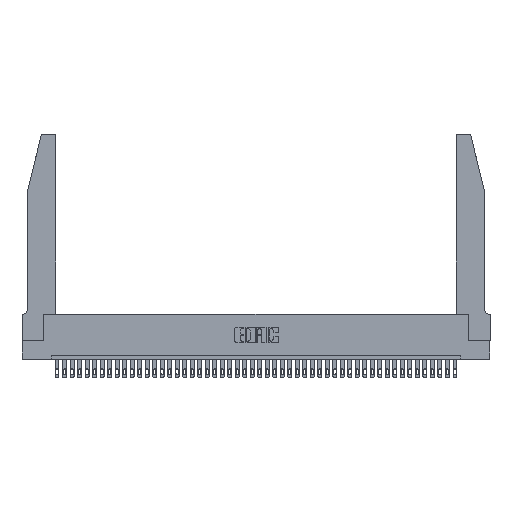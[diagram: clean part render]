
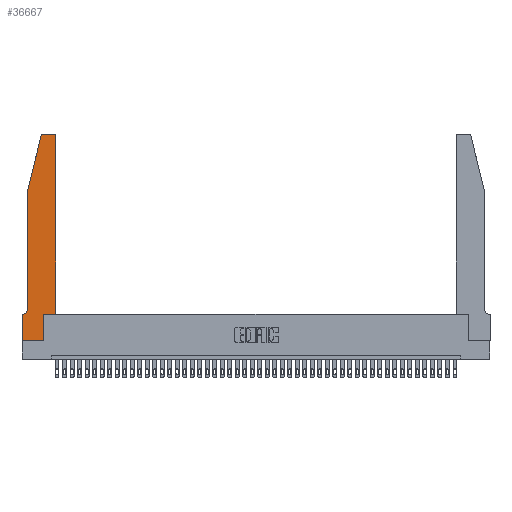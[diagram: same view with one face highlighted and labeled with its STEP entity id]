
A CAD part, top view. The second image highlights one B-rep face of the part: STEP entity #36667.
In plain terms, the highlighted planar face has unit normal (0, 0, 1).
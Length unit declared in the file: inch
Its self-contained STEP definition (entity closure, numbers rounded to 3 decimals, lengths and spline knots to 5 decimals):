
#34 = LINE ( 'NONE', #6574, #41725 ) ;
#71 = LINE ( 'NONE', #24568, #39164 ) ;
#725 = DIRECTION ( 'NONE',  ( 0., 1., 0. ) ) ;
#2326 = LINE ( 'NONE', #5138, #9770 ) ;
#2414 = EDGE_CURVE ( 'NONE', #17838, #34856, #2326, .T. ) ;
#3315 = ORIENTED_EDGE ( 'NONE', *, *, #34419, .T. ) ;
#3596 = VERTEX_POINT ( 'NONE', #22459 ) ;
#3743 = EDGE_CURVE ( 'NONE', #11515, #40789, #71, .T. ) ;
#4116 = EDGE_CURVE ( 'NONE', #7840, #17838, #31760, .T. ) ;
#4780 = VECTOR ( 'NONE', #27494, 39.37008 ) ;
#5112 = ORIENTED_EDGE ( 'NONE', *, *, #27863, .T. ) ;
#5138 = CARTESIAN_POINT ( 'NONE',  ( 0.0755, 2., 0.37 ) ) ;
#5243 = CARTESIAN_POINT ( 'NONE',  ( 0., 0., 0.37 ) ) ;
#5890 = CARTESIAN_POINT ( 'NONE',  ( 0., 0., 0.37 ) ) ;
#6040 = EDGE_CURVE ( 'NONE', #40789, #29439, #8405, .T. ) ;
#6149 = AXIS2_PLACEMENT_3D ( 'NONE', #17358, #23974, #27797 ) ;
#6574 = CARTESIAN_POINT ( 'NONE',  ( 0.4505, 0.35, 0.37 ) ) ;
#6720 = ORIENTED_EDGE ( 'NONE', *, *, #4116, .T. ) ;
#7116 = FACE_OUTER_BOUND ( 'NONE', #42128, .T. ) ;
#7541 = CARTESIAN_POINT ( 'NONE',  ( 0.2865, 0.35, 0.37 ) ) ;
#7772 = DIRECTION ( 'NONE',  ( 0., -1., 0. ) ) ;
#7806 = DIRECTION ( 'NONE',  ( 1., 0., 0. ) ) ;
#7840 = VERTEX_POINT ( 'NONE', #15061 ) ;
#7943 = CARTESIAN_POINT ( 'NONE',  ( 0.4205, 2.72, 0.37 ) ) ;
#8077 = LINE ( 'NONE', #31076, #24962 ) ;
#8382 = VERTEX_POINT ( 'NONE', #7541 ) ;
#8405 = LINE ( 'NONE', #5243, #33708 ) ;
#9770 = VECTOR ( 'NONE', #29033, 39.37008 ) ;
#9802 = ORIENTED_EDGE ( 'NONE', *, *, #6040, .T. ) ;
#10179 = CARTESIAN_POINT ( 'NONE',  ( 0.0755, 0.42, 0.37 ) ) ;
#10533 = CARTESIAN_POINT ( 'NONE',  ( 0.0755, 2., 0.37 ) ) ;
#11062 = DIRECTION ( 'NONE',  ( -1., 0., 0. ) ) ;
#11515 = VERTEX_POINT ( 'NONE', #38339 ) ;
#12745 = LINE ( 'NONE', #27349, #4780 ) ;
#13095 = DIRECTION ( 'NONE',  ( 1., 0., 0. ) ) ;
#14653 = CARTESIAN_POINT ( 'NONE',  ( 0.2865, 0.35, 0.37 ) ) ;
#15061 = CARTESIAN_POINT ( 'NONE',  ( 0.25487, 2.72718, 0.37 ) ) ;
#15376 = VECTOR ( 'NONE', #24355, 39.37008 ) ;
#15972 = DIRECTION ( 'NONE',  ( 0., 0., 1. ) ) ;
#16013 = CIRCLE ( 'NONE', #38579, 0.03 ) ;
#16124 = PLANE ( 'NONE',  #16844 ) ;
#16266 = ORIENTED_EDGE ( 'NONE', *, *, #16835, .T. ) ;
#16835 = EDGE_CURVE ( 'NONE', #3596, #7840, #31516, .T. ) ;
#16844 = AXIS2_PLACEMENT_3D ( 'NONE', #39666, #15972, #43043 ) ;
#17358 = CARTESIAN_POINT ( 'NONE',  ( 0.284, 2.72, 0.37 ) ) ;
#17789 = VERTEX_POINT ( 'NONE', #37803 ) ;
#17838 = VERTEX_POINT ( 'NONE', #10533 ) ;
#18339 = ORIENTED_EDGE ( 'NONE', *, *, #2414, .T. ) ;
#19147 = LINE ( 'NONE', #42747, #26560 ) ;
#20956 = CIRCLE ( 'NONE', #36287, 0.07 ) ;
#21856 = EDGE_CURVE ( 'NONE', #39464, #23357, #12745, .T. ) ;
#22459 = CARTESIAN_POINT ( 'NONE',  ( 0.284, 2.75, 0.37 ) ) ;
#23357 = VERTEX_POINT ( 'NONE', #32208 ) ;
#23974 = DIRECTION ( 'NONE',  ( 0., 0., 1. ) ) ;
#24355 = DIRECTION ( 'NONE',  ( -0.239, -0.971, 0. ) ) ;
#24568 = CARTESIAN_POINT ( 'NONE',  ( 0., 0., 0.37 ) ) ;
#24962 = VECTOR ( 'NONE', #11062, 39.37008 ) ;
#25328 = ORIENTED_EDGE ( 'NONE', *, *, #31943, .T. ) ;
#25417 = VERTEX_POINT ( 'NONE', #39149 ) ;
#25497 = DIRECTION ( 'NONE',  ( 1., 0., 0. ) ) ;
#26364 = EDGE_CURVE ( 'NONE', #23357, #25417, #16013, .T. ) ;
#26424 = CARTESIAN_POINT ( 'NONE',  ( 0.4505, 0.35, 0.37 ) ) ;
#26560 = VECTOR ( 'NONE', #36134, 39.37008 ) ;
#27349 = CARTESIAN_POINT ( 'NONE',  ( 0.4505, 0.35, 0.37 ) ) ;
#27494 = DIRECTION ( 'NONE',  ( 0., 1., 0. ) ) ;
#27797 = DIRECTION ( 'NONE',  ( 1., 0., 0. ) ) ;
#27863 = EDGE_CURVE ( 'NONE', #8382, #39464, #34, .T. ) ;
#28119 = ORIENTED_EDGE ( 'NONE', *, *, #21856, .T. ) ;
#28754 = ORIENTED_EDGE ( 'NONE', *, *, #32165, .T. ) ;
#28892 = DIRECTION ( 'NONE',  ( 0., 0., -1. ) ) ;
#29033 = DIRECTION ( 'NONE',  ( 0., -1., 0. ) ) ;
#29439 = VERTEX_POINT ( 'NONE', #34916 ) ;
#31076 = CARTESIAN_POINT ( 'NONE',  ( 0.0755, 0.35, 0.37 ) ) ;
#31516 = CIRCLE ( 'NONE', #6149, 0.03 ) ;
#31760 = LINE ( 'NONE', #40867, #15376 ) ;
#31826 = DIRECTION ( 'NONE',  ( 0., 0., 1. ) ) ;
#31943 = EDGE_CURVE ( 'NONE', #17789, #11515, #8077, .T. ) ;
#32165 = EDGE_CURVE ( 'NONE', #25417, #3596, #19147, .T. ) ;
#32208 = CARTESIAN_POINT ( 'NONE',  ( 0.4505, 2.72, 0.37 ) ) ;
#32255 = DIRECTION ( 'NONE',  ( -1., 0., 0. ) ) ;
#33708 = VECTOR ( 'NONE', #25497, 39.37008 ) ;
#34419 = EDGE_CURVE ( 'NONE', #29439, #8382, #35798, .T. ) ;
#34856 = VERTEX_POINT ( 'NONE', #10179 ) ;
#34916 = CARTESIAN_POINT ( 'NONE',  ( 0.2865, 0., 0.37 ) ) ;
#35198 = EDGE_CURVE ( 'NONE', #34856, #17789, #20956, .T. ) ;
#35534 = ORIENTED_EDGE ( 'NONE', *, *, #3743, .T. ) ;
#35798 = LINE ( 'NONE', #14653, #40499 ) ;
#35813 = CARTESIAN_POINT ( 'NONE',  ( 0.0055, 0.42, 0.37 ) ) ;
#36134 = DIRECTION ( 'NONE',  ( -1., 0., 0. ) ) ;
#36287 = AXIS2_PLACEMENT_3D ( 'NONE', #35813, #28892, #32255 ) ;
#36667 = ADVANCED_FACE ( 'NONE', ( #7116 ), #16124, .T. ) ;
#37803 = CARTESIAN_POINT ( 'NONE',  ( 0.0055, 0.35, 0.37 ) ) ;
#38339 = CARTESIAN_POINT ( 'NONE',  ( 0., 0.35, 0.37 ) ) ;
#38579 = AXIS2_PLACEMENT_3D ( 'NONE', #7943, #31826, #7806 ) ;
#39149 = CARTESIAN_POINT ( 'NONE',  ( 0.4205, 2.75, 0.37 ) ) ;
#39164 = VECTOR ( 'NONE', #7772, 39.37008 ) ;
#39464 = VERTEX_POINT ( 'NONE', #26424 ) ;
#39666 = CARTESIAN_POINT ( 'NONE',  ( 0., 0.35, 0.37 ) ) ;
#40499 = VECTOR ( 'NONE', #725, 39.37008 ) ;
#40789 = VERTEX_POINT ( 'NONE', #5890 ) ;
#40867 = CARTESIAN_POINT ( 'NONE',  ( 0.0755, 2., 0.37 ) ) ;
#41372 = ORIENTED_EDGE ( 'NONE', *, *, #26364, .T. ) ;
#41725 = VECTOR ( 'NONE', #13095, 39.37008 ) ;
#42128 = EDGE_LOOP ( 'NONE', ( #28754, #16266, #6720, #18339, #43735, #25328, #35534, #9802, #3315, #5112, #28119, #41372 ) ) ;
#42747 = CARTESIAN_POINT ( 'NONE',  ( 0.2605, 2.75, 0.37 ) ) ;
#43043 = DIRECTION ( 'NONE',  ( 1., 0., 0. ) ) ;
#43735 = ORIENTED_EDGE ( 'NONE', *, *, #35198, .T. ) ;
